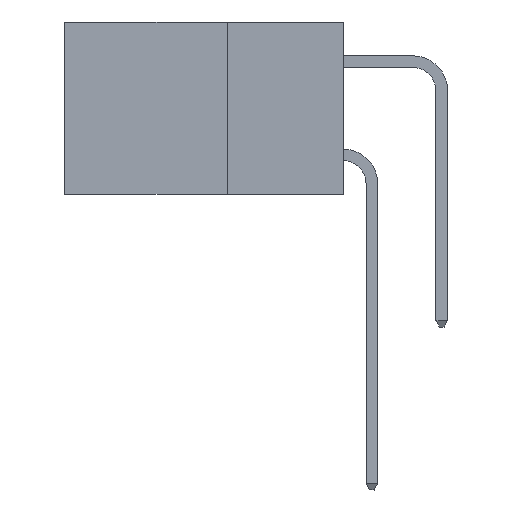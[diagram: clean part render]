
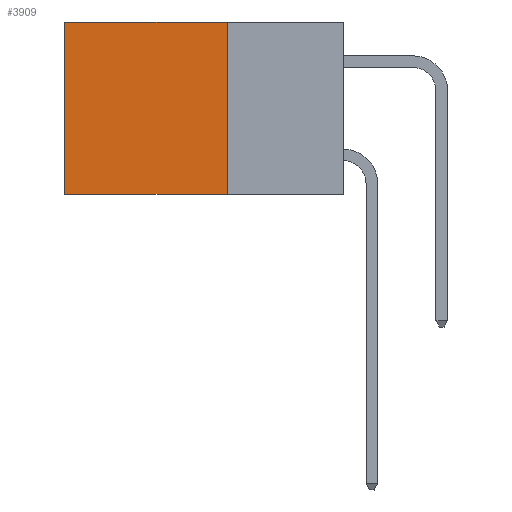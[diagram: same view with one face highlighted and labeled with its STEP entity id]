
A CAD part, left-side view. The second image highlights one B-rep face of the part: STEP entity #3909.
In plain terms, the highlighted planar face has unit normal (-1, 0, 0).
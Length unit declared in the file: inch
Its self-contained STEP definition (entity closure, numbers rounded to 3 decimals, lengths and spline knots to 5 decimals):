
#573 = DIRECTION ( 'NONE',  ( 0., 0., -1. ) ) ;
#875 = LINE ( 'NONE', #7414, #6803 ) ;
#1224 = FACE_OUTER_BOUND ( 'NONE', #17213, .T. ) ;
#1273 = ORIENTED_EDGE ( 'NONE', *, *, #6589, .F. ) ;
#1799 = DIRECTION ( 'NONE',  ( 0., 0., -1. ) ) ;
#3400 = LINE ( 'NONE', #4895, #5733 ) ;
#3909 = ADVANCED_FACE ( 'NONE', ( #1224 ), #19089, .F. ) ;
#4165 = EDGE_CURVE ( 'NONE', #13039, #13734, #11630, .T. ) ;
#4449 = DIRECTION ( 'NONE',  ( 0., 0., -1. ) ) ;
#4895 = CARTESIAN_POINT ( 'NONE',  ( 0.2615, 0.25, -0.37 ) ) ;
#5140 = CARTESIAN_POINT ( 'NONE',  ( 0.2615, 0.6, -0.37 ) ) ;
#5281 = CARTESIAN_POINT ( 'NONE',  ( 0.2615, 0.25, 0. ) ) ;
#5387 = EDGE_CURVE ( 'NONE', #7784, #13039, #14512, .T. ) ;
#5733 = VECTOR ( 'NONE', #1799, 39.37008 ) ;
#6589 = EDGE_CURVE ( 'NONE', #17514, #13734, #875, .T. ) ;
#6803 = VECTOR ( 'NONE', #14253, 39.37008 ) ;
#7414 = CARTESIAN_POINT ( 'NONE',  ( 0.2615, 0.25, -0.37 ) ) ;
#7771 = DIRECTION ( 'NONE',  ( 1., 0., 0. ) ) ;
#7784 = VERTEX_POINT ( 'NONE', #5281 ) ;
#8743 = CARTESIAN_POINT ( 'NONE',  ( 0.2615, 0.25, -0.37 ) ) ;
#8872 = CARTESIAN_POINT ( 'NONE',  ( 0.2615, 0.6, 0. ) ) ;
#9247 = VECTOR ( 'NONE', #573, 39.37008 ) ;
#11623 = AXIS2_PLACEMENT_3D ( 'NONE', #17089, #7771, #4449 ) ;
#11630 = LINE ( 'NONE', #18235, #9247 ) ;
#13039 = VERTEX_POINT ( 'NONE', #8872 ) ;
#13734 = VERTEX_POINT ( 'NONE', #5140 ) ;
#13829 = ORIENTED_EDGE ( 'NONE', *, *, #4165, .T. ) ;
#13903 = ORIENTED_EDGE ( 'NONE', *, *, #17060, .F. ) ;
#14253 = DIRECTION ( 'NONE',  ( 0., 1., 0. ) ) ;
#14512 = LINE ( 'NONE', #19613, #21007 ) ;
#14832 = DIRECTION ( 'NONE',  ( 0., 1., 0. ) ) ;
#17060 = EDGE_CURVE ( 'NONE', #7784, #17514, #3400, .T. ) ;
#17089 = CARTESIAN_POINT ( 'NONE',  ( 0.2615, 0.25, -0.37 ) ) ;
#17213 = EDGE_LOOP ( 'NONE', ( #13829, #1273, #13903, #19621 ) ) ;
#17514 = VERTEX_POINT ( 'NONE', #8743 ) ;
#18235 = CARTESIAN_POINT ( 'NONE',  ( 0.2615, 0.6, -0.37 ) ) ;
#19089 = PLANE ( 'NONE',  #11623 ) ;
#19613 = CARTESIAN_POINT ( 'NONE',  ( 0.2615, 0.25, 0. ) ) ;
#19621 = ORIENTED_EDGE ( 'NONE', *, *, #5387, .T. ) ;
#21007 = VECTOR ( 'NONE', #14832, 39.37008 ) ;
